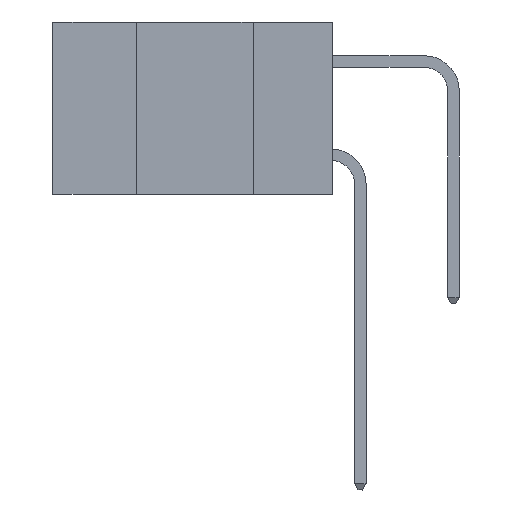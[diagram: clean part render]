
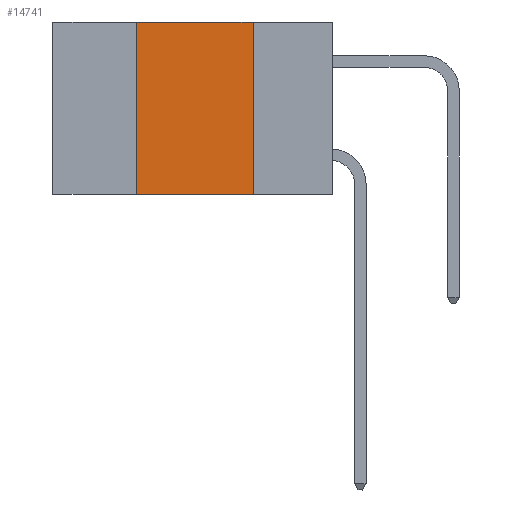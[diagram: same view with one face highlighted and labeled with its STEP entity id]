
A CAD part, left-side view. The second image highlights one B-rep face of the part: STEP entity #14741.
In plain terms, the highlighted planar face has unit normal (-1, 0, 0).
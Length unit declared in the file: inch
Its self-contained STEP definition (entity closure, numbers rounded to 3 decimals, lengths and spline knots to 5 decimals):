
#148 = LINE ( 'NONE', #6121, #16222 ) ;
#450 = AXIS2_PLACEMENT_3D ( 'NONE', #31639, #28893, #29222 ) ;
#3327 = DIRECTION ( 'NONE',  ( 0., 0., -1. ) ) ;
#3368 = CARTESIAN_POINT ( 'NONE',  ( 0., 0.42, 0. ) ) ;
#5955 = LINE ( 'NONE', #12582, #15351 ) ;
#6121 = CARTESIAN_POINT ( 'NONE',  ( 0., 0.6, 0. ) ) ;
#8434 = DIRECTION ( 'NONE',  ( 0., -1., 0. ) ) ;
#8478 = CARTESIAN_POINT ( 'NONE',  ( 0., 0.17, 0. ) ) ;
#8752 = EDGE_LOOP ( 'NONE', ( #25906, #10700, #15418, #10450 ) ) ;
#10450 = ORIENTED_EDGE ( 'NONE', *, *, #27869, .T. ) ;
#10700 = ORIENTED_EDGE ( 'NONE', *, *, #25907, .F. ) ;
#12582 = CARTESIAN_POINT ( 'NONE',  ( 0., 0.6, -0.37 ) ) ;
#14200 = CARTESIAN_POINT ( 'NONE',  ( 0., 0.17, 0. ) ) ;
#14739 = VERTEX_POINT ( 'NONE', #26481 ) ;
#14741 = ADVANCED_FACE ( 'NONE', ( #18764 ), #31535, .F. ) ;
#15091 = DIRECTION ( 'NONE',  ( 0., -1., 0. ) ) ;
#15168 = VECTOR ( 'NONE', #15522, 39.37008 ) ;
#15351 = VECTOR ( 'NONE', #15091, 39.37008 ) ;
#15418 = ORIENTED_EDGE ( 'NONE', *, *, #30753, .F. ) ;
#15522 = DIRECTION ( 'NONE',  ( 0., 0., 1. ) ) ;
#16222 = VECTOR ( 'NONE', #8434, 39.37008 ) ;
#17493 = EDGE_CURVE ( 'NONE', #20692, #14739, #19394, .T. ) ;
#17863 = CARTESIAN_POINT ( 'NONE',  ( 0., 0.42, -0.37 ) ) ;
#18067 = CARTESIAN_POINT ( 'NONE',  ( 0., 0.42, 0. ) ) ;
#18764 = FACE_OUTER_BOUND ( 'NONE', #8752, .T. ) ;
#19394 = LINE ( 'NONE', #8478, #23704 ) ;
#20692 = VERTEX_POINT ( 'NONE', #14200 ) ;
#21366 = VERTEX_POINT ( 'NONE', #17863 ) ;
#22610 = LINE ( 'NONE', #3368, #15168 ) ;
#23272 = VERTEX_POINT ( 'NONE', #18067 ) ;
#23704 = VECTOR ( 'NONE', #3327, 39.37008 ) ;
#25906 = ORIENTED_EDGE ( 'NONE', *, *, #17493, .F. ) ;
#25907 = EDGE_CURVE ( 'NONE', #23272, #20692, #148, .T. ) ;
#26481 = CARTESIAN_POINT ( 'NONE',  ( 0., 0.17, -0.37 ) ) ;
#27869 = EDGE_CURVE ( 'NONE', #21366, #14739, #5955, .T. ) ;
#28893 = DIRECTION ( 'NONE',  ( 1., 0., 0. ) ) ;
#29222 = DIRECTION ( 'NONE',  ( 0., 0., -1. ) ) ;
#30753 = EDGE_CURVE ( 'NONE', #21366, #23272, #22610, .T. ) ;
#31535 = PLANE ( 'NONE',  #450 ) ;
#31639 = CARTESIAN_POINT ( 'NONE',  ( 0., 0.6, 0. ) ) ;
